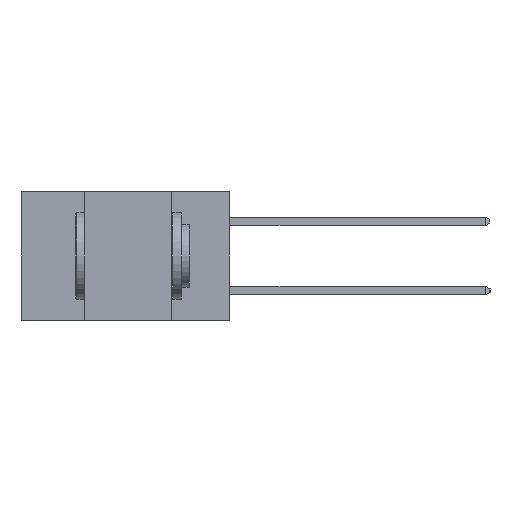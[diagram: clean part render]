
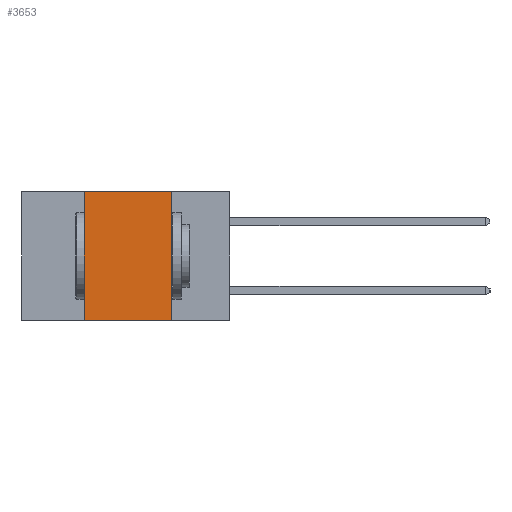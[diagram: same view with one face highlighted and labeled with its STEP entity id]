
A CAD part, left-side view. The second image highlights one B-rep face of the part: STEP entity #3653.
In plain terms, the highlighted planar face has unit normal (-1, 0, 0).
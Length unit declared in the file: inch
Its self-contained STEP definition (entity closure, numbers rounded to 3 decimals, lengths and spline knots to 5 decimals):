
#184 = ORIENTED_EDGE ( 'NONE', *, *, #5133, .F. ) ;
#675 = VECTOR ( 'NONE', #7209, 39.37008 ) ;
#917 = CARTESIAN_POINT ( 'NONE',  ( 0., 0.6, 0. ) ) ;
#949 = DIRECTION ( 'NONE',  ( 0., -1., 0. ) ) ;
#2258 = CARTESIAN_POINT ( 'NONE',  ( 0., 0.17, -0.37 ) ) ;
#2290 = ORIENTED_EDGE ( 'NONE', *, *, #12478, .F. ) ;
#2356 = DIRECTION ( 'NONE',  ( 0., 0., 1. ) ) ;
#2985 = VERTEX_POINT ( 'NONE', #6910 ) ;
#3559 = DIRECTION ( 'NONE',  ( 0., -1., 0. ) ) ;
#3605 = CARTESIAN_POINT ( 'NONE',  ( 0., 0.6, -0.37 ) ) ;
#3653 = ADVANCED_FACE ( 'NONE', ( #7753 ), #14921, .F. ) ;
#3826 = VERTEX_POINT ( 'NONE', #12691 ) ;
#3833 = ORIENTED_EDGE ( 'NONE', *, *, #14422, .F. ) ;
#4234 = VECTOR ( 'NONE', #3559, 39.37008 ) ;
#4814 = EDGE_CURVE ( 'NONE', #2985, #15644, #14373, .T. ) ;
#5133 = EDGE_CURVE ( 'NONE', #8801, #3826, #13018, .T. ) ;
#5179 = AXIS2_PLACEMENT_3D ( 'NONE', #14818, #14791, #14759 ) ;
#6152 = VECTOR ( 'NONE', #949, 39.37008 ) ;
#6910 = CARTESIAN_POINT ( 'NONE',  ( 0., 0.42, -0.37 ) ) ;
#7209 = DIRECTION ( 'NONE',  ( 0., 0., -1. ) ) ;
#7753 = FACE_OUTER_BOUND ( 'NONE', #9321, .T. ) ;
#8498 = CARTESIAN_POINT ( 'NONE',  ( 0., 0.42, -0.37 ) ) ;
#8640 = CARTESIAN_POINT ( 'NONE',  ( 0., 0.42, 0. ) ) ;
#8801 = VERTEX_POINT ( 'NONE', #8640 ) ;
#9321 = EDGE_LOOP ( 'NONE', ( #3833, #184, #2290, #13589 ) ) ;
#9730 = CARTESIAN_POINT ( 'NONE',  ( 0., 0.17, -0.37 ) ) ;
#10467 = LINE ( 'NONE', #2258, #675 ) ;
#11649 = VECTOR ( 'NONE', #2356, 39.37008 ) ;
#12478 = EDGE_CURVE ( 'NONE', #2985, #8801, #14919, .T. ) ;
#12691 = CARTESIAN_POINT ( 'NONE',  ( 0., 0.17, 0. ) ) ;
#13018 = LINE ( 'NONE', #917, #6152 ) ;
#13589 = ORIENTED_EDGE ( 'NONE', *, *, #4814, .T. ) ;
#14373 = LINE ( 'NONE', #3605, #4234 ) ;
#14422 = EDGE_CURVE ( 'NONE', #3826, #15644, #10467, .T. ) ;
#14759 = DIRECTION ( 'NONE',  ( 0., 0., -1. ) ) ;
#14791 = DIRECTION ( 'NONE',  ( 1., 0., 0. ) ) ;
#14818 = CARTESIAN_POINT ( 'NONE',  ( 0., 0.6, 0. ) ) ;
#14919 = LINE ( 'NONE', #8498, #11649 ) ;
#14921 = PLANE ( 'NONE',  #5179 ) ;
#15644 = VERTEX_POINT ( 'NONE', #9730 ) ;
